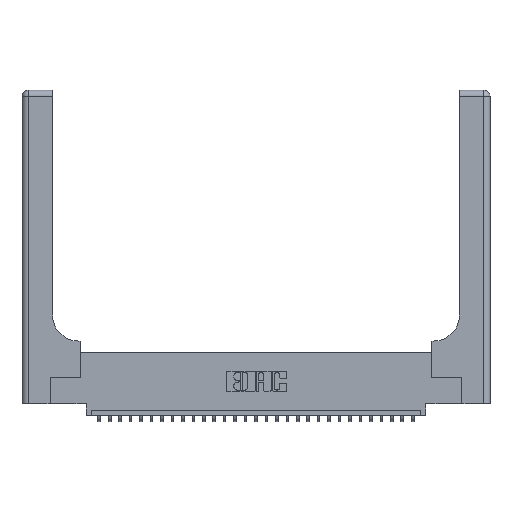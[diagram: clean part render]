
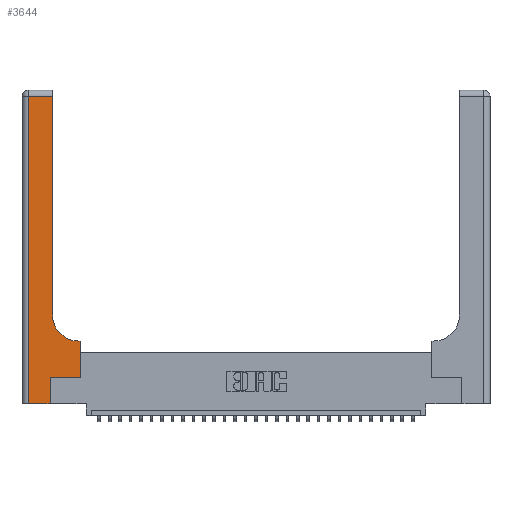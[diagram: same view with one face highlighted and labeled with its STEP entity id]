
A CAD part, top view. The second image highlights one B-rep face of the part: STEP entity #3644.
In plain terms, the highlighted planar face has unit normal (0, 0, 1).
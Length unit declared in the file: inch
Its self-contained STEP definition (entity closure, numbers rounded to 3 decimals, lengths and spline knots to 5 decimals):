
#210 = CARTESIAN_POINT ( 'NONE',  ( 0.5415, 0.6, 0.37 ) ) ;
#796 = LINE ( 'NONE', #28356, #14738 ) ;
#1429 = EDGE_CURVE ( 'NONE', #2275, #9472, #796, .T. ) ;
#2114 = CARTESIAN_POINT ( 'NONE',  ( 0.5585, 0.25, 0.37 ) ) ;
#2216 = DIRECTION ( 'NONE',  ( 0., 1., 0. ) ) ;
#2275 = VERTEX_POINT ( 'NONE', #19966 ) ;
#2453 = EDGE_LOOP ( 'NONE', ( #18599, #17562, #11819, #14665, #19173, #17713, #13146, #10800, #19584 ) ) ;
#2506 = DIRECTION ( 'NONE',  ( 0., -1., 0. ) ) ;
#3636 = CARTESIAN_POINT ( 'NONE',  ( 0., 2.94, 0.37 ) ) ;
#3644 = ADVANCED_FACE ( 'NONE', ( #26117 ), #18326, .F. ) ;
#3712 = EDGE_CURVE ( 'NONE', #9245, #29587, #18124, .T. ) ;
#4541 = EDGE_CURVE ( 'NONE', #28098, #22573, #30008, .T. ) ;
#5931 = VECTOR ( 'NONE', #22685, 39.37008 ) ;
#6313 = CARTESIAN_POINT ( 'NONE',  ( 0.2915, 3., 0.37 ) ) ;
#6333 = VECTOR ( 'NONE', #15777, 39.37008 ) ;
#6488 = DIRECTION ( 'NONE',  ( 0., 0., -1. ) ) ;
#7062 = AXIS2_PLACEMENT_3D ( 'NONE', #16265, #20469, #22816 ) ;
#7520 = LINE ( 'NONE', #6313, #6333 ) ;
#8751 = CARTESIAN_POINT ( 'NONE',  ( 0., 0., 0.37 ) ) ;
#8853 = CARTESIAN_POINT ( 'NONE',  ( 0.2915, 2.94, 0.37 ) ) ;
#9245 = VERTEX_POINT ( 'NONE', #20639 ) ;
#9472 = VERTEX_POINT ( 'NONE', #23868 ) ;
#10800 = ORIENTED_EDGE ( 'NONE', *, *, #4541, .T. ) ;
#11161 = AXIS2_PLACEMENT_3D ( 'NONE', #23081, #6488, #27553 ) ;
#11819 = ORIENTED_EDGE ( 'NONE', *, *, #3712, .T. ) ;
#13085 = VECTOR ( 'NONE', #29467, 39.37008 ) ;
#13146 = ORIENTED_EDGE ( 'NONE', *, *, #15855, .T. ) ;
#13224 = VECTOR ( 'NONE', #20385, 39.37008 ) ;
#14263 = EDGE_CURVE ( 'NONE', #19217, #9245, #29702, .T. ) ;
#14665 = ORIENTED_EDGE ( 'NONE', *, *, #19203, .T. ) ;
#14699 = VERTEX_POINT ( 'NONE', #16735 ) ;
#14738 = VECTOR ( 'NONE', #17164, 39.37008 ) ;
#15724 = EDGE_CURVE ( 'NONE', #14699, #19217, #7520, .T. ) ;
#15777 = DIRECTION ( 'NONE',  ( 0., 1., 0. ) ) ;
#15855 = EDGE_CURVE ( 'NONE', #24642, #28098, #20560, .T. ) ;
#16265 = CARTESIAN_POINT ( 'NONE',  ( 0., 3., 0.37 ) ) ;
#16357 = CIRCLE ( 'NONE', #11161, 0.25 ) ;
#16558 = CARTESIAN_POINT ( 'NONE',  ( 0.06, 3., 0.37 ) ) ;
#16635 = VECTOR ( 'NONE', #2506, 39.37008 ) ;
#16735 = CARTESIAN_POINT ( 'NONE',  ( 0.2915, 0.85, 0.37 ) ) ;
#17164 = DIRECTION ( 'NONE',  ( 0., 1., 0. ) ) ;
#17562 = ORIENTED_EDGE ( 'NONE', *, *, #14263, .T. ) ;
#17713 = ORIENTED_EDGE ( 'NONE', *, *, #27419, .T. ) ;
#18088 = VECTOR ( 'NONE', #19835, 39.37008 ) ;
#18124 = LINE ( 'NONE', #16558, #16635 ) ;
#18326 = PLANE ( 'NONE',  #7062 ) ;
#18599 = ORIENTED_EDGE ( 'NONE', *, *, #15724, .T. ) ;
#19173 = ORIENTED_EDGE ( 'NONE', *, *, #1429, .T. ) ;
#19203 = EDGE_CURVE ( 'NONE', #29587, #2275, #28010, .T. ) ;
#19217 = VERTEX_POINT ( 'NONE', #8853 ) ;
#19438 = LINE ( 'NONE', #25170, #13224 ) ;
#19584 = ORIENTED_EDGE ( 'NONE', *, *, #23446, .T. ) ;
#19835 = DIRECTION ( 'NONE',  ( -1., 0., 0. ) ) ;
#19966 = CARTESIAN_POINT ( 'NONE',  ( 0.269, 0., 0.37 ) ) ;
#20385 = DIRECTION ( 'NONE',  ( 1., 0., 0. ) ) ;
#20469 = DIRECTION ( 'NONE',  ( 0., 0., -1. ) ) ;
#20560 = LINE ( 'NONE', #21056, #24198 ) ;
#20639 = CARTESIAN_POINT ( 'NONE',  ( 0.06, 2.94, 0.37 ) ) ;
#21056 = CARTESIAN_POINT ( 'NONE',  ( 0.5585, 0.25, 0.37 ) ) ;
#21264 = CARTESIAN_POINT ( 'NONE',  ( 0.06, 0., 0.37 ) ) ;
#22573 = VERTEX_POINT ( 'NONE', #210 ) ;
#22685 = DIRECTION ( 'NONE',  ( -1., 0., 0. ) ) ;
#22816 = DIRECTION ( 'NONE',  ( -1., 0., 0. ) ) ;
#23081 = CARTESIAN_POINT ( 'NONE',  ( 0.5415, 0.85, 0.37 ) ) ;
#23446 = EDGE_CURVE ( 'NONE', #22573, #14699, #16357, .T. ) ;
#23868 = CARTESIAN_POINT ( 'NONE',  ( 0.269, 0.25, 0.37 ) ) ;
#24198 = VECTOR ( 'NONE', #2216, 39.37008 ) ;
#24642 = VERTEX_POINT ( 'NONE', #2114 ) ;
#25170 = CARTESIAN_POINT ( 'NONE',  ( 0.269, 0.25, 0.37 ) ) ;
#25724 = CARTESIAN_POINT ( 'NONE',  ( 0.2915, 0.6, 0.37 ) ) ;
#26117 = FACE_OUTER_BOUND ( 'NONE', #2453, .T. ) ;
#27419 = EDGE_CURVE ( 'NONE', #9472, #24642, #19438, .T. ) ;
#27441 = CARTESIAN_POINT ( 'NONE',  ( 0.5585, 0.6, 0.37 ) ) ;
#27553 = DIRECTION ( 'NONE',  ( 1., 0., 0. ) ) ;
#28010 = LINE ( 'NONE', #8751, #13085 ) ;
#28098 = VERTEX_POINT ( 'NONE', #27441 ) ;
#28356 = CARTESIAN_POINT ( 'NONE',  ( 0.269, 0., 0.37 ) ) ;
#29467 = DIRECTION ( 'NONE',  ( 1., 0., 0. ) ) ;
#29587 = VERTEX_POINT ( 'NONE', #21264 ) ;
#29702 = LINE ( 'NONE', #3636, #18088 ) ;
#30008 = LINE ( 'NONE', #25724, #5931 ) ;
